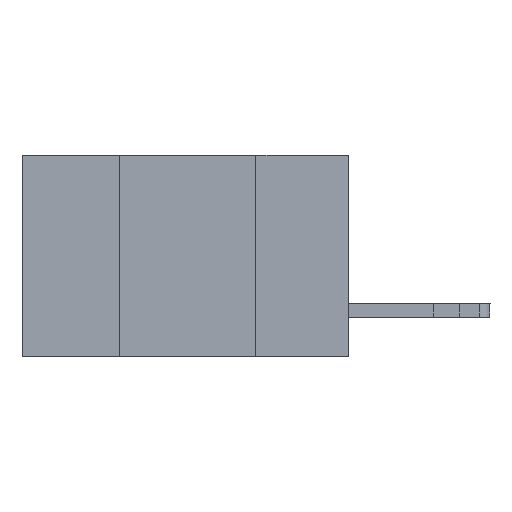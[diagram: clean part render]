
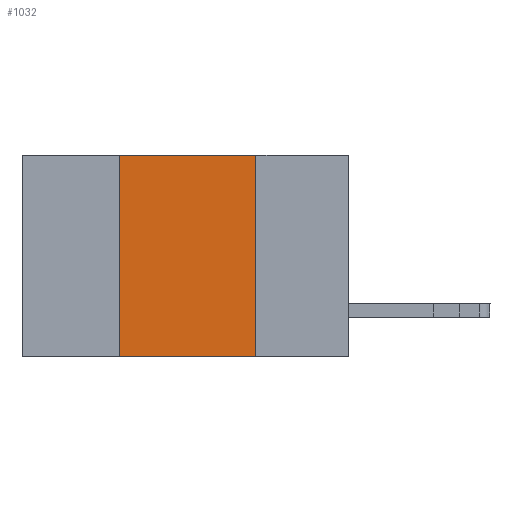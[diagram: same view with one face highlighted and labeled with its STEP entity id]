
A CAD part, left-side view. The second image highlights one B-rep face of the part: STEP entity #1032.
In plain terms, the highlighted planar face has unit normal (-1, 0, 0).
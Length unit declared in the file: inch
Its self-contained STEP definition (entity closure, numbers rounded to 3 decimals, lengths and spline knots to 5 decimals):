
#308 = DIRECTION ( 'NONE',  ( 0., -1., 0. ) ) ;
#557 = DIRECTION ( 'NONE',  ( 1., 0., 0. ) ) ;
#794 = LINE ( 'NONE', #13134, #11558 ) ;
#1032 = ADVANCED_FACE ( 'NONE', ( #12736 ), #7909, .F. ) ;
#1616 = DIRECTION ( 'NONE',  ( 0., 0., -1. ) ) ;
#1622 = LINE ( 'NONE', #12670, #4021 ) ;
#1863 = CARTESIAN_POINT ( 'NONE',  ( 0., 0.6, 0. ) ) ;
#2804 = CARTESIAN_POINT ( 'NONE',  ( 0., 0.6, -0.37 ) ) ;
#3886 = CARTESIAN_POINT ( 'NONE',  ( 0., 0.6, 0. ) ) ;
#4021 = VECTOR ( 'NONE', #6699, 39.37008 ) ;
#4418 = VERTEX_POINT ( 'NONE', #13045 ) ;
#5007 = ORIENTED_EDGE ( 'NONE', *, *, #7854, .T. ) ;
#5074 = AXIS2_PLACEMENT_3D ( 'NONE', #1863, #557, #1616 ) ;
#5270 = ORIENTED_EDGE ( 'NONE', *, *, #7029, .F. ) ;
#5714 = DIRECTION ( 'NONE',  ( 0., 0., -1. ) ) ;
#5784 = EDGE_LOOP ( 'NONE', ( #5270, #7089, #12348, #5007 ) ) ;
#6699 = DIRECTION ( 'NONE',  ( 0., 0., 1. ) ) ;
#7029 = EDGE_CURVE ( 'NONE', #9286, #13988, #794, .T. ) ;
#7089 = ORIENTED_EDGE ( 'NONE', *, *, #10041, .F. ) ;
#7446 = VERTEX_POINT ( 'NONE', #12952 ) ;
#7461 = DIRECTION ( 'NONE',  ( 0., -1., 0. ) ) ;
#7854 = EDGE_CURVE ( 'NONE', #4418, #13988, #10184, .T. ) ;
#7909 = PLANE ( 'NONE',  #5074 ) ;
#8496 = EDGE_CURVE ( 'NONE', #4418, #7446, #1622, .T. ) ;
#8934 = VECTOR ( 'NONE', #308, 39.37008 ) ;
#8983 = CARTESIAN_POINT ( 'NONE',  ( 0., 0.17, 0. ) ) ;
#9286 = VERTEX_POINT ( 'NONE', #8983 ) ;
#9831 = LINE ( 'NONE', #3886, #8934 ) ;
#10041 = EDGE_CURVE ( 'NONE', #7446, #9286, #9831, .T. ) ;
#10184 = LINE ( 'NONE', #2804, #11457 ) ;
#11457 = VECTOR ( 'NONE', #7461, 39.37008 ) ;
#11558 = VECTOR ( 'NONE', #5714, 39.37008 ) ;
#12348 = ORIENTED_EDGE ( 'NONE', *, *, #8496, .F. ) ;
#12670 = CARTESIAN_POINT ( 'NONE',  ( 0., 0.42, 0. ) ) ;
#12736 = FACE_OUTER_BOUND ( 'NONE', #5784, .T. ) ;
#12952 = CARTESIAN_POINT ( 'NONE',  ( 0., 0.42, 0. ) ) ;
#13045 = CARTESIAN_POINT ( 'NONE',  ( 0., 0.42, -0.37 ) ) ;
#13091 = CARTESIAN_POINT ( 'NONE',  ( 0., 0.17, -0.37 ) ) ;
#13134 = CARTESIAN_POINT ( 'NONE',  ( 0., 0.17, 0. ) ) ;
#13988 = VERTEX_POINT ( 'NONE', #13091 ) ;
